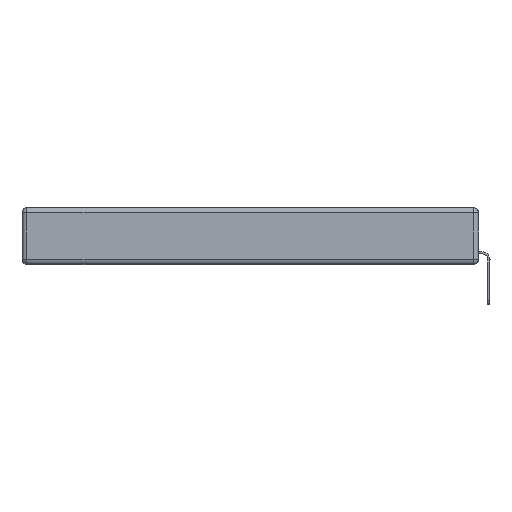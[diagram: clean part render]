
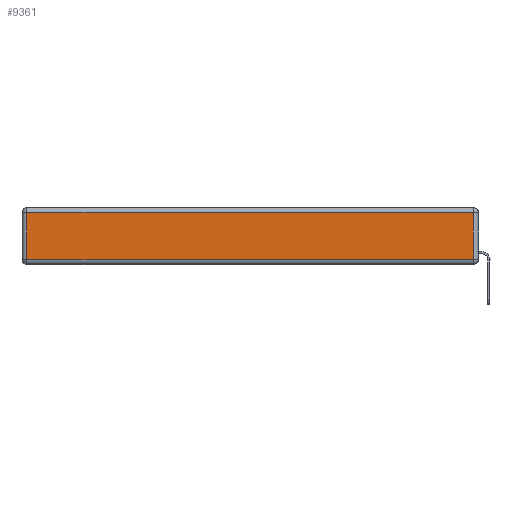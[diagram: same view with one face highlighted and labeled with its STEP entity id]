
A CAD part, left-side view. The second image highlights one B-rep face of the part: STEP entity #9361.
In plain terms, the highlighted planar face has unit normal (-1, 0, 0).
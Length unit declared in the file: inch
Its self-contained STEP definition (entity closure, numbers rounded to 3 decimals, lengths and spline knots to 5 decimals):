
#523 = EDGE_CURVE ( 'NONE', #12163, #9268, #532, .T. ) ;
#532 = LINE ( 'NONE', #10821, #3803 ) ;
#581 = FACE_OUTER_BOUND ( 'NONE', #11642, .T. ) ;
#648 = DIRECTION ( 'NONE',  ( 0., 0., 1. ) ) ;
#1056 = DIRECTION ( 'NONE',  ( 0., 1., 0. ) ) ;
#1349 = EDGE_CURVE ( 'NONE', #9268, #5632, #7642, .T. ) ;
#1830 = DIRECTION ( 'NONE',  ( 0., -1., 0. ) ) ;
#3801 = CARTESIAN_POINT ( 'NONE',  ( 0., 2.72, -0.313 ) ) ;
#3803 = VECTOR ( 'NONE', #1830, 39.37008 ) ;
#3815 = DIRECTION ( 'NONE',  ( 0., 0., 1. ) ) ;
#3838 = VECTOR ( 'NONE', #3815, 39.37008 ) ;
#4167 = ORIENTED_EDGE ( 'NONE', *, *, #9854, .T. ) ;
#5242 = PLANE ( 'NONE',  #14410 ) ;
#5632 = VERTEX_POINT ( 'NONE', #9297 ) ;
#6081 = CARTESIAN_POINT ( 'NONE',  ( 0., 0.03, -0.313 ) ) ;
#6556 = VERTEX_POINT ( 'NONE', #11629 ) ;
#6735 = VECTOR ( 'NONE', #9868, 39.37008 ) ;
#7384 = CARTESIAN_POINT ( 'NONE',  ( 0., 0.03, -0.343 ) ) ;
#7642 = LINE ( 'NONE', #7384, #3838 ) ;
#9252 = ORIENTED_EDGE ( 'NONE', *, *, #1349, .T. ) ;
#9268 = VERTEX_POINT ( 'NONE', #6081 ) ;
#9297 = CARTESIAN_POINT ( 'NONE',  ( 0., 0.03, -0.03 ) ) ;
#9361 = ADVANCED_FACE ( 'NONE', ( #581 ), #5242, .T. ) ;
#9854 = EDGE_CURVE ( 'NONE', #5632, #6556, #14543, .T. ) ;
#9868 = DIRECTION ( 'NONE',  ( 0., 0., -1. ) ) ;
#9916 = EDGE_CURVE ( 'NONE', #6556, #12163, #10099, .T. ) ;
#10099 = LINE ( 'NONE', #13349, #6735 ) ;
#10338 = ORIENTED_EDGE ( 'NONE', *, *, #523, .T. ) ;
#10821 = CARTESIAN_POINT ( 'NONE',  ( 0., 0., -0.313 ) ) ;
#10921 = CARTESIAN_POINT ( 'NONE',  ( 0., 2.75, -0.03 ) ) ;
#11629 = CARTESIAN_POINT ( 'NONE',  ( 0., 2.72, -0.03 ) ) ;
#11642 = EDGE_LOOP ( 'NONE', ( #10338, #9252, #4167, #13636 ) ) ;
#11832 = CARTESIAN_POINT ( 'NONE',  ( 0., 0., -0.343 ) ) ;
#12037 = DIRECTION ( 'NONE',  ( -1., 0., 0. ) ) ;
#12163 = VERTEX_POINT ( 'NONE', #3801 ) ;
#13349 = CARTESIAN_POINT ( 'NONE',  ( 0., 2.72, -0.343 ) ) ;
#13636 = ORIENTED_EDGE ( 'NONE', *, *, #9916, .T. ) ;
#14281 = VECTOR ( 'NONE', #1056, 39.37008 ) ;
#14410 = AXIS2_PLACEMENT_3D ( 'NONE', #11832, #12037, #648 ) ;
#14543 = LINE ( 'NONE', #10921, #14281 ) ;
